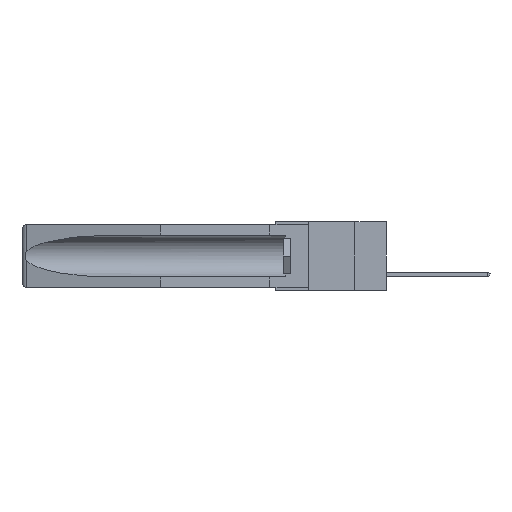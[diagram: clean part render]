
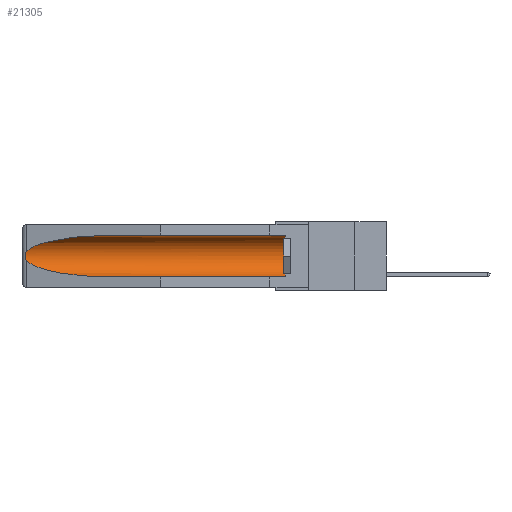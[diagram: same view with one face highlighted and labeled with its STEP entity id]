
A CAD part, left-side view. The second image highlights one B-rep face of the part: STEP entity #21305.
In plain terms, the highlighted cylindrical face has radius 2.857 mm (diameter 5.715 mm), a partial arc.
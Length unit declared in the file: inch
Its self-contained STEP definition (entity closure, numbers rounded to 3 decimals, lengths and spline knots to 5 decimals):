
#182 = CARTESIAN_POINT ( 'NONE',  ( 0.26597, 1.52961, -0.15275 ) ) ;
#309 = ORIENTED_EDGE ( 'NONE', *, *, #5182, .T. ) ;
#454 = CARTESIAN_POINT ( 'NONE',  ( 0.26537, 1.52718, -0.14972 ) ) ;
#636 = CARTESIAN_POINT ( 'NONE',  ( 0.26537, 1.52718, -0.19328 ) ) ;
#800 = CARTESIAN_POINT ( 'NONE',  ( 0.26537, 1.52718, -0.14972 ) ) ;
#1066 = ORIENTED_EDGE ( 'NONE', *, *, #21488, .T. ) ;
#1488 = EDGE_CURVE ( 'NONE', #22644, #2627, #13449, .T. ) ;
#1560 = CARTESIAN_POINT ( 'NONE',  ( 0.2675, 1.53308, -0.16763 ) ) ;
#1585 = CARTESIAN_POINT ( 'NONE',  ( 0.26537, 1.52718, -0.19328 ) ) ;
#1630 = CARTESIAN_POINT ( 'NONE',  ( 0.155, -0.30754, -0.1715 ) ) ;
#1724 = ORIENTED_EDGE ( 'NONE', *, *, #2251, .F. ) ;
#1834 = DIRECTION ( 'NONE',  ( 0., 0., 1. ) ) ;
#2251 = EDGE_CURVE ( 'NONE', #22644, #9908, #15957, .T. ) ;
#2627 = VERTEX_POINT ( 'NONE', #9275 ) ;
#2897 = CARTESIAN_POINT ( 'NONE',  ( 0.21114, 1.30732, -0.284 ) ) ;
#3654 = DIRECTION ( 'NONE',  ( 0., 0., 1. ) ) ;
#3912 =( BOUNDED_CURVE ( )  B_SPLINE_CURVE ( 3, ( #17006, #20933, #25015, #8995 ),
 .UNSPECIFIED., .F., .T. ) 
 B_SPLINE_CURVE_WITH_KNOTS ( ( 4, 4 ),
 ( 4.71239, 6.08839 ),
 .UNSPECIFIED. ) 
 CURVE ( )  GEOMETRIC_REPRESENTATION_ITEM ( )  RATIONAL_B_SPLINE_CURVE ( ( 1., 0.848, 0.848, 1. ) ) 
 REPRESENTATION_ITEM ( '' )  );
#4380 =( BOUNDED_CURVE ( )  B_SPLINE_CURVE ( 3, ( #636, #6663, #2897, #22997 ),
 .UNSPECIFIED., .F., .F. ) 
 B_SPLINE_CURVE_WITH_KNOTS ( ( 4, 4 ),
 ( 0.1948, 1.5708 ),
 .UNSPECIFIED. ) 
 CURVE ( )  GEOMETRIC_REPRESENTATION_ITEM ( )  RATIONAL_B_SPLINE_CURVE ( ( 1., 0.848, 0.848, 1. ) ) 
 REPRESENTATION_ITEM ( '' )  );
#4392 = CARTESIAN_POINT ( 'NONE',  ( 0.26597, 1.5296, -0.19026 ) ) ;
#4520 = CARTESIAN_POINT ( 'NONE',  ( 0.155, 0.126, -0.284 ) ) ;
#5182 = EDGE_CURVE ( 'NONE', #24461, #23275, #3912, .T. ) ;
#5439 = DIRECTION ( 'NONE',  ( 0., 1., 0. ) ) ;
#5790 = CARTESIAN_POINT ( 'NONE',  ( 0.155, 0.126, -0.1715 ) ) ;
#6475 = CARTESIAN_POINT ( 'NONE',  ( 0.26537, 1.52718, -0.19328 ) ) ;
#6663 = CARTESIAN_POINT ( 'NONE',  ( 0.25451, 1.48313, -0.24835 ) ) ;
#6666 = FACE_OUTER_BOUND ( 'NONE', #15044, .T. ) ;
#6934 = AXIS2_PLACEMENT_3D ( 'NONE', #1630, #15572, #3654 ) ;
#7115 = ORIENTED_EDGE ( 'NONE', *, *, #15015, .T. ) ;
#8995 = CARTESIAN_POINT ( 'NONE',  ( 0.26537, 1.52718, -0.14972 ) ) ;
#9275 = CARTESIAN_POINT ( 'NONE',  ( 0.155, 0.126, -0.059 ) ) ;
#9583 = CARTESIAN_POINT ( 'NONE',  ( 0.2673, 1.53269, -0.17917 ) ) ;
#9908 = VERTEX_POINT ( 'NONE', #25594 ) ;
#10011 = CARTESIAN_POINT ( 'NONE',  ( 0.26655, 1.53094, -0.18657 ) ) ;
#11923 = VECTOR ( 'NONE', #5439, 39.37008 ) ;
#13449 = CIRCLE ( 'NONE', #22149, 0.1125 ) ;
#13509 = CYLINDRICAL_SURFACE ( 'NONE', #6934, 0.1125 ) ;
#13645 = B_SPLINE_CURVE_WITH_KNOTS ( 'NONE', 3,
 ( #454, #182, #23435, #21517, #1560, #17534, #9583, #10011, #4392, #6475 ),
 .UNSPECIFIED., .F., .F.,
 ( 4, 2, 2, 2, 4 ),
 ( 0., 0.00029, 0.00058, 0.00087, 0.00117 ),
 .UNSPECIFIED. ) ;
#13791 = VECTOR ( 'NONE', #18192, 39.37008 ) ;
#14145 = EDGE_CURVE ( 'NONE', #23275, #20458, #13645, .T. ) ;
#15015 = EDGE_CURVE ( 'NONE', #20458, #9908, #4380, .T. ) ;
#15044 = EDGE_LOOP ( 'NONE', ( #309, #20758, #7115, #1724, #23355, #1066 ) ) ;
#15572 = DIRECTION ( 'NONE',  ( 0., 1., 0. ) ) ;
#15686 = CARTESIAN_POINT ( 'NONE',  ( 0.155, -0.30754, -0.059 ) ) ;
#15957 = LINE ( 'NONE', #19941, #13791 ) ;
#17006 = CARTESIAN_POINT ( 'NONE',  ( 0.155, 1.07973, -0.059 ) ) ;
#17534 = CARTESIAN_POINT ( 'NONE',  ( 0.2675, 1.53308, -0.17534 ) ) ;
#17638 = DIRECTION ( 'NONE',  ( 0., -1., 0. ) ) ;
#18192 = DIRECTION ( 'NONE',  ( 0., 1., 0. ) ) ;
#19941 = CARTESIAN_POINT ( 'NONE',  ( 0.155, -0.30754, -0.284 ) ) ;
#20458 = VERTEX_POINT ( 'NONE', #1585 ) ;
#20758 = ORIENTED_EDGE ( 'NONE', *, *, #14145, .T. ) ;
#20933 = CARTESIAN_POINT ( 'NONE',  ( 0.21114, 1.30732, -0.059 ) ) ;
#21305 = ADVANCED_FACE ( 'NONE', ( #6666 ), #13509, .F. ) ;
#21488 = EDGE_CURVE ( 'NONE', #2627, #24461, #25342, .T. ) ;
#21517 = CARTESIAN_POINT ( 'NONE',  ( 0.2673, 1.5327, -0.16383 ) ) ;
#22149 = AXIS2_PLACEMENT_3D ( 'NONE', #5790, #17638, #1834 ) ;
#22536 = CARTESIAN_POINT ( 'NONE',  ( 0.155, 1.07973, -0.059 ) ) ;
#22644 = VERTEX_POINT ( 'NONE', #4520 ) ;
#22997 = CARTESIAN_POINT ( 'NONE',  ( 0.155, 1.07973, -0.284 ) ) ;
#23275 = VERTEX_POINT ( 'NONE', #800 ) ;
#23355 = ORIENTED_EDGE ( 'NONE', *, *, #1488, .T. ) ;
#23435 = CARTESIAN_POINT ( 'NONE',  ( 0.26654, 1.53092, -0.15636 ) ) ;
#24461 = VERTEX_POINT ( 'NONE', #22536 ) ;
#25015 = CARTESIAN_POINT ( 'NONE',  ( 0.25451, 1.48313, -0.09465 ) ) ;
#25342 = LINE ( 'NONE', #15686, #11923 ) ;
#25594 = CARTESIAN_POINT ( 'NONE',  ( 0.155, 1.07973, -0.284 ) ) ;
